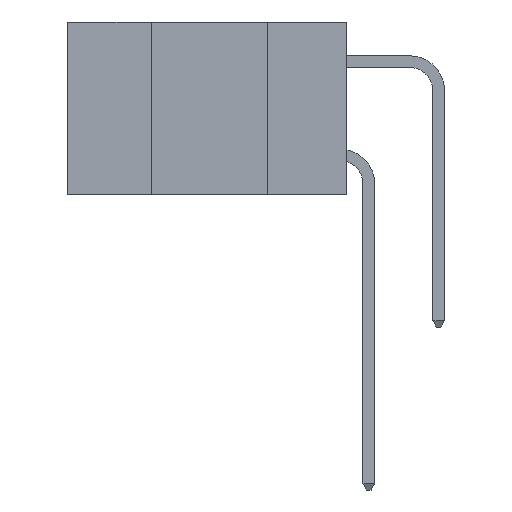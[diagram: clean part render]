
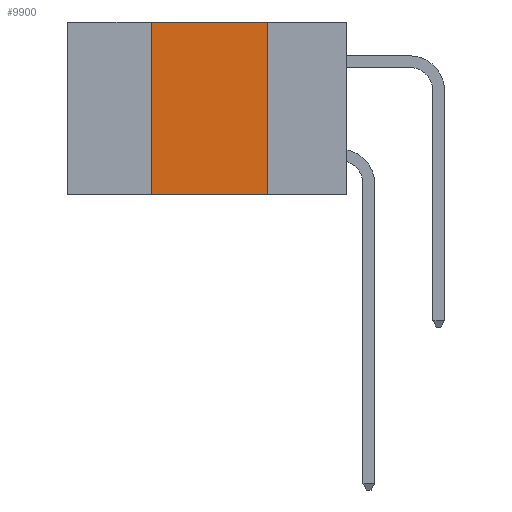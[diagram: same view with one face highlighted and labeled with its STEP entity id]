
A CAD part, left-side view. The second image highlights one B-rep face of the part: STEP entity #9900.
In plain terms, the highlighted planar face has unit normal (-1, 0, 0).
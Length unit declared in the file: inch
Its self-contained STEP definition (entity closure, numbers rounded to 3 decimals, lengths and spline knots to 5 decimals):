
#60 = VECTOR ( 'NONE', #3766, 39.37008 ) ;
#217 = LINE ( 'NONE', #6742, #21683 ) ;
#743 = DIRECTION ( 'NONE',  ( 1., 0., 0. ) ) ;
#1500 = EDGE_CURVE ( 'NONE', #5536, #11190, #18975, .T. ) ;
#2172 = EDGE_CURVE ( 'NONE', #5536, #7020, #7847, .T. ) ;
#2422 = AXIS2_PLACEMENT_3D ( 'NONE', #11140, #743, #25753 ) ;
#2526 = DIRECTION ( 'NONE',  ( 0., -1., 0. ) ) ;
#3766 = DIRECTION ( 'NONE',  ( 0., 0., 1. ) ) ;
#5536 = VERTEX_POINT ( 'NONE', #16539 ) ;
#6475 = ORIENTED_EDGE ( 'NONE', *, *, #24648, .F. ) ;
#6742 = CARTESIAN_POINT ( 'NONE',  ( 0., 0.6, 0. ) ) ;
#7020 = VERTEX_POINT ( 'NONE', #13741 ) ;
#7581 = CARTESIAN_POINT ( 'NONE',  ( 0., 0.6, -0.37 ) ) ;
#7793 = CARTESIAN_POINT ( 'NONE',  ( 0., 0.17, 0. ) ) ;
#7847 = LINE ( 'NONE', #12055, #60 ) ;
#9638 = CARTESIAN_POINT ( 'NONE',  ( 0., 0.17, -0.37 ) ) ;
#9900 = ADVANCED_FACE ( 'NONE', ( #20388 ), #13219, .F. ) ;
#11140 = CARTESIAN_POINT ( 'NONE',  ( 0., 0.6, 0. ) ) ;
#11190 = VERTEX_POINT ( 'NONE', #9638 ) ;
#11199 = VERTEX_POINT ( 'NONE', #24093 ) ;
#12055 = CARTESIAN_POINT ( 'NONE',  ( 0., 0.42, 0. ) ) ;
#13219 = PLANE ( 'NONE',  #2422 ) ;
#13741 = CARTESIAN_POINT ( 'NONE',  ( 0., 0.42, 0. ) ) ;
#15033 = ORIENTED_EDGE ( 'NONE', *, *, #25674, .F. ) ;
#15946 = VECTOR ( 'NONE', #15959, 39.37008 ) ;
#15959 = DIRECTION ( 'NONE',  ( 0., 0., -1. ) ) ;
#16539 = CARTESIAN_POINT ( 'NONE',  ( 0., 0.42, -0.37 ) ) ;
#17647 = DIRECTION ( 'NONE',  ( 0., -1., 0. ) ) ;
#18975 = LINE ( 'NONE', #7581, #23537 ) ;
#20388 = FACE_OUTER_BOUND ( 'NONE', #23272, .T. ) ;
#21417 = LINE ( 'NONE', #7793, #15946 ) ;
#21683 = VECTOR ( 'NONE', #2526, 39.37008 ) ;
#23272 = EDGE_LOOP ( 'NONE', ( #6475, #15033, #26313, #26274 ) ) ;
#23537 = VECTOR ( 'NONE', #17647, 39.37008 ) ;
#24093 = CARTESIAN_POINT ( 'NONE',  ( 0., 0.17, 0. ) ) ;
#24648 = EDGE_CURVE ( 'NONE', #11199, #11190, #21417, .T. ) ;
#25674 = EDGE_CURVE ( 'NONE', #7020, #11199, #217, .T. ) ;
#25753 = DIRECTION ( 'NONE',  ( 0., 0., -1. ) ) ;
#26274 = ORIENTED_EDGE ( 'NONE', *, *, #1500, .T. ) ;
#26313 = ORIENTED_EDGE ( 'NONE', *, *, #2172, .F. ) ;
